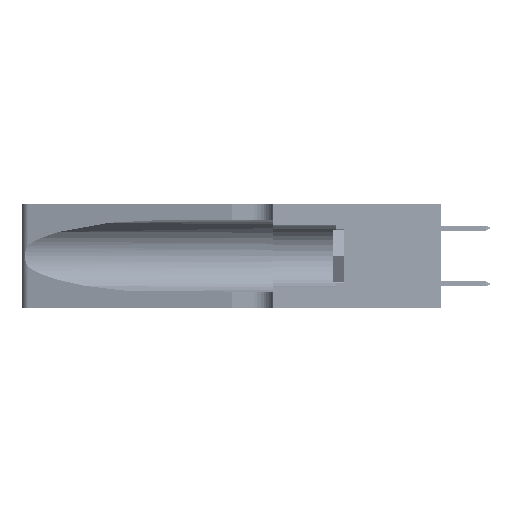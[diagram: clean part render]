
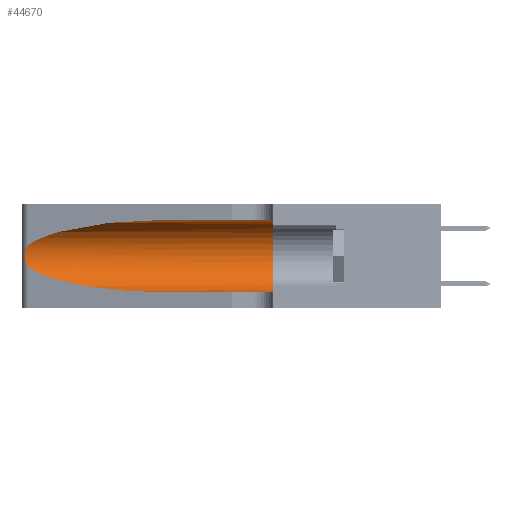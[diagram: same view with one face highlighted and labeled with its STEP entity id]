
A CAD part, left-side view. The second image highlights one B-rep face of the part: STEP entity #44670.
In plain terms, the highlighted cylindrical face has radius 3.308 mm (diameter 6.617 mm), a partial arc.
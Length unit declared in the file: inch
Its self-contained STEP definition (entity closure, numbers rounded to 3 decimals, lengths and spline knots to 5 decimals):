
#56 = CARTESIAN_POINT ( 'NONE',  ( 0.1305, 0.72297, 0.05475 ) ) ;
#331 = CARTESIAN_POINT ( 'NONE',  ( 0.1305, 0.72297, 0.31525 ) ) ;
#477 = CARTESIAN_POINT ( 'NONE',  ( 0.25487, 1.22718, 0.22369 ) ) ;
#2391 = CARTESIAN_POINT ( 'NONE',  ( 0.1305, 0.72297, 0.31525 ) ) ;
#4104 = DIRECTION ( 'NONE',  ( 0., 1., 0. ) ) ;
#4527 = ORIENTED_EDGE ( 'NONE', *, *, #39798, .T. ) ;
#4551 = VERTEX_POINT ( 'NONE', #477 ) ;
#5172 = CARTESIAN_POINT ( 'NONE',  ( 0.25487, 1.22718, 0.22369 ) ) ;
#6199 = VECTOR ( 'NONE', #10053, 39.37008 ) ;
#6452 = VERTEX_POINT ( 'NONE', #331 ) ;
#9776 = CARTESIAN_POINT ( 'NONE',  ( 0.18966, 0.96281, 0.31525 ) ) ;
#10053 = DIRECTION ( 'NONE',  ( 0., -1., 0. ) ) ;
#10111 = CARTESIAN_POINT ( 'NONE',  ( 0.26017, 1.23833, 0.17102 ) ) ;
#11004 = EDGE_LOOP ( 'NONE', ( #4527, #39487, #46086, #14404, #25186, #42205 ) ) ;
#11129 = CARTESIAN_POINT ( 'NONE',  ( 0.18966, 0.96281, 0.05475 ) ) ;
#12730 =( BOUNDED_CURVE ( )  B_SPLINE_CURVE ( 3, ( #2391, #9776, #27851, #31970 ),
 .UNSPECIFIED., .F., .T. ) 
 B_SPLINE_CURVE_WITH_KNOTS ( ( 4, 4 ),
 ( 1.5708, 2.84003 ),
 .UNSPECIFIED. ) 
 CURVE ( )  GEOMETRIC_REPRESENTATION_ITEM ( )  RATIONAL_B_SPLINE_CURVE ( ( 1., 0.87, 0.87, 1. ) ) 
 REPRESENTATION_ITEM ( '' )  );
#12774 = LINE ( 'NONE', #20586, #27764 ) ;
#13790 = DIRECTION ( 'NONE',  ( 0., -1., 0. ) ) ;
#13990 = CARTESIAN_POINT ( 'NONE',  ( 0.25854, 1.2359, 0.20912 ) ) ;
#14404 = ORIENTED_EDGE ( 'NONE', *, *, #26932, .T. ) ;
#15059 = VERTEX_POINT ( 'NONE', #47338 ) ;
#15137 = EDGE_CURVE ( 'NONE', #43600, #15059, #46386, .T. ) ;
#16953 = DIRECTION ( 'NONE',  ( 0., 0., -1. ) ) ;
#17735 = CARTESIAN_POINT ( 'NONE',  ( 0.25787, 1.23484, 0.2124 ) ) ;
#17910 = CARTESIAN_POINT ( 'NONE',  ( 0.1305, 0.72297, 0.05475 ) ) ;
#18482 = DIRECTION ( 'NONE',  ( 0., 0., 1. ) ) ;
#18734 = CARTESIAN_POINT ( 'NONE',  ( 0.2373, 1.15595, 0.08982 ) ) ;
#20479 = CARTESIAN_POINT ( 'NONE',  ( 0.1305, 1.61858, 0.185 ) ) ;
#20586 = CARTESIAN_POINT ( 'NONE',  ( 0.1305, 1.61858, 0.31525 ) ) ;
#20929 = CARTESIAN_POINT ( 'NONE',  ( 0.26075, 1.23896, 0.19203 ) ) ;
#21418 = CARTESIAN_POINT ( 'NONE',  ( 0.25555, 1.22993, 0.14849 ) ) ;
#23203 = AXIS2_PLACEMENT_3D ( 'NONE', #20479, #38896, #16953 ) ;
#24617 = CARTESIAN_POINT ( 'NONE',  ( 0.25639, 1.23186, 0.15144 ) ) ;
#24835 =( BOUNDED_CURVE ( )  B_SPLINE_CURVE ( 3, ( #28890, #18734, #11129, #56 ),
 .UNSPECIFIED., .F., .T. ) 
 B_SPLINE_CURVE_WITH_KNOTS ( ( 4, 4 ),
 ( 3.44316, 4.71239 ),
 .UNSPECIFIED. ) 
 CURVE ( )  GEOMETRIC_REPRESENTATION_ITEM ( )  RATIONAL_B_SPLINE_CURVE ( ( 1., 0.87, 0.87, 1. ) ) 
 REPRESENTATION_ITEM ( '' )  );
#25186 = ORIENTED_EDGE ( 'NONE', *, *, #15137, .F. ) ;
#25378 = EDGE_CURVE ( 'NONE', #6452, #43600, #12774, .T. ) ;
#25659 = CARTESIAN_POINT ( 'NONE',  ( 0.1305, 0.35, 0.31525 ) ) ;
#26932 = EDGE_CURVE ( 'NONE', #46619, #15059, #35493, .T. ) ;
#27764 = VECTOR ( 'NONE', #13790, 39.37008 ) ;
#27806 = B_SPLINE_CURVE_WITH_KNOTS ( 'NONE', 3,
 ( #5172, #38247, #46919, #17735, #13990, #31834, #20929, #46609, #10111, #39665, #39039, #24617, #21418, #32157 ),
 .UNSPECIFIED., .F., .F.,
 ( 4, 2, 2, 2, 2, 2, 4 ),
 ( 0., 0.00027, 0.00053, 0.00107, 0.0016, 0.00187, 0.00214 ),
 .UNSPECIFIED. ) ;
#27851 = CARTESIAN_POINT ( 'NONE',  ( 0.2373, 1.15595, 0.28018 ) ) ;
#28890 = CARTESIAN_POINT ( 'NONE',  ( 0.25487, 1.22718, 0.14631 ) ) ;
#31834 = CARTESIAN_POINT ( 'NONE',  ( 0.26018, 1.23835, 0.19895 ) ) ;
#31970 = CARTESIAN_POINT ( 'NONE',  ( 0.25487, 1.22718, 0.22369 ) ) ;
#32157 = CARTESIAN_POINT ( 'NONE',  ( 0.25487, 1.22718, 0.14631 ) ) ;
#33050 = EDGE_CURVE ( 'NONE', #34959, #46619, #24835, .T. ) ;
#33822 = AXIS2_PLACEMENT_3D ( 'NONE', #40869, #4104, #18482 ) ;
#34959 = VERTEX_POINT ( 'NONE', #40183 ) ;
#35493 = LINE ( 'NONE', #46704, #6199 ) ;
#36265 = EDGE_CURVE ( 'NONE', #4551, #34959, #27806, .T. ) ;
#38247 = CARTESIAN_POINT ( 'NONE',  ( 0.25555, 1.22994, 0.2215 ) ) ;
#38896 = DIRECTION ( 'NONE',  ( 0., -1., 0. ) ) ;
#39039 = CARTESIAN_POINT ( 'NONE',  ( 0.25789, 1.23486, 0.15765 ) ) ;
#39487 = ORIENTED_EDGE ( 'NONE', *, *, #36265, .T. ) ;
#39665 = CARTESIAN_POINT ( 'NONE',  ( 0.25856, 1.23593, 0.16098 ) ) ;
#39798 = EDGE_CURVE ( 'NONE', #6452, #4551, #12730, .T. ) ;
#40183 = CARTESIAN_POINT ( 'NONE',  ( 0.25487, 1.22718, 0.14631 ) ) ;
#40869 = CARTESIAN_POINT ( 'NONE',  ( 0.1305, 0.35, 0.185 ) ) ;
#42205 = ORIENTED_EDGE ( 'NONE', *, *, #25378, .F. ) ;
#43206 = FACE_OUTER_BOUND ( 'NONE', #11004, .T. ) ;
#43600 = VERTEX_POINT ( 'NONE', #25659 ) ;
#44371 = CYLINDRICAL_SURFACE ( 'NONE', #23203, 0.13025 ) ;
#44670 = ADVANCED_FACE ( 'NONE', ( #43206 ), #44371, .F. ) ;
#46086 = ORIENTED_EDGE ( 'NONE', *, *, #33050, .T. ) ;
#46386 = CIRCLE ( 'NONE', #33822, 0.13025 ) ;
#46609 = CARTESIAN_POINT ( 'NONE',  ( 0.26075, 1.23896, 0.178 ) ) ;
#46619 = VERTEX_POINT ( 'NONE', #17910 ) ;
#46704 = CARTESIAN_POINT ( 'NONE',  ( 0.1305, 1.61858, 0.05475 ) ) ;
#46919 = CARTESIAN_POINT ( 'NONE',  ( 0.25639, 1.23184, 0.21858 ) ) ;
#47338 = CARTESIAN_POINT ( 'NONE',  ( 0.1305, 0.35, 0.05475 ) ) ;
